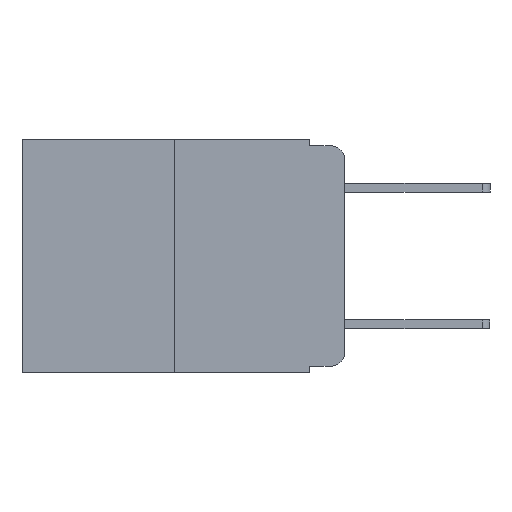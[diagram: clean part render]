
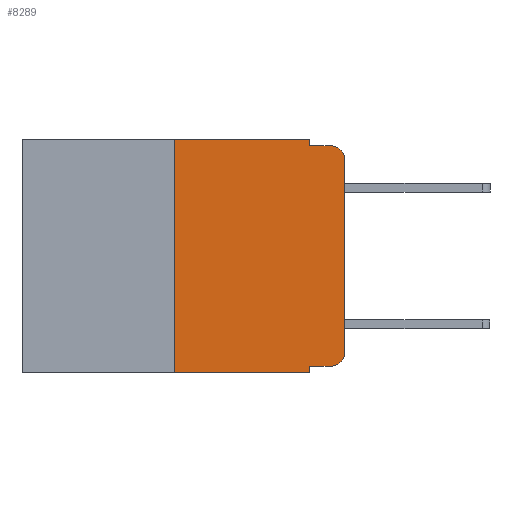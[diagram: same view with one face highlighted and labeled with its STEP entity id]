
A CAD part, left-side view. The second image highlights one B-rep face of the part: STEP entity #8289.
In plain terms, the highlighted planar face has unit normal (-1, 0, 0).
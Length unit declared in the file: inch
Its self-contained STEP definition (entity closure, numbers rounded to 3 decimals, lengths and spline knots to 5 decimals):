
#242 = EDGE_CURVE ( 'NONE', #3376, #22150, #15281, .T. ) ;
#620 = CARTESIAN_POINT ( 'NONE',  ( 0., 0.02, -0.01 ) ) ;
#632 = VECTOR ( 'NONE', #13422, 39.37008 ) ;
#712 = AXIS2_PLACEMENT_3D ( 'NONE', #9768, #23434, #2373 ) ;
#1002 = ORIENTED_EDGE ( 'NONE', *, *, #242, .F. ) ;
#1067 = VECTOR ( 'NONE', #6610, 39.37008 ) ;
#1385 = DIRECTION ( 'NONE',  ( 1., 0., 0. ) ) ;
#2243 = ORIENTED_EDGE ( 'NONE', *, *, #25216, .F. ) ;
#2373 = DIRECTION ( 'NONE',  ( 0., 0., -1. ) ) ;
#2882 = EDGE_CURVE ( 'NONE', #5389, #16315, #20441, .T. ) ;
#3294 = CARTESIAN_POINT ( 'NONE',  ( 0., 0., 0. ) ) ;
#3376 = VERTEX_POINT ( 'NONE', #22678 ) ;
#3440 = EDGE_CURVE ( 'NONE', #22150, #9264, #23692, .T. ) ;
#4256 = CARTESIAN_POINT ( 'NONE',  ( 0., 0.051, -0.343 ) ) ;
#4480 = CARTESIAN_POINT ( 'NONE',  ( 0., 0.02, -0.333 ) ) ;
#4535 = DIRECTION ( 'NONE',  ( -1., 0., 0. ) ) ;
#4758 = VECTOR ( 'NONE', #19102, 39.37008 ) ;
#5281 = DIRECTION ( 'NONE',  ( 0., 0., 1. ) ) ;
#5389 = VERTEX_POINT ( 'NONE', #19181 ) ;
#5987 = VECTOR ( 'NONE', #5281, 39.37008 ) ;
#6610 = DIRECTION ( 'NONE',  ( 0., -1., 0. ) ) ;
#6726 = AXIS2_PLACEMENT_3D ( 'NONE', #11439, #1385, #10585 ) ;
#6978 = LINE ( 'NONE', #20381, #1067 ) ;
#7067 = EDGE_CURVE ( 'NONE', #21983, #12084, #20606, .T. ) ;
#7747 = VECTOR ( 'NONE', #15739, 39.37008 ) ;
#8142 = EDGE_LOOP ( 'NONE', ( #10676, #12561, #14055, #14674, #1002, #2243, #24409, #10335, #13502, #14078 ) ) ;
#8289 = ADVANCED_FACE ( 'NONE', ( #14418 ), #19187, .F. ) ;
#8391 = CARTESIAN_POINT ( 'NONE',  ( 0., 0.25, 0. ) ) ;
#8671 = EDGE_CURVE ( 'NONE', #25123, #18181, #6978, .T. ) ;
#8984 = AXIS2_PLACEMENT_3D ( 'NONE', #16349, #4535, #18314 ) ;
#9008 = CARTESIAN_POINT ( 'NONE',  ( 0., 0.473, -0.343 ) ) ;
#9264 = VERTEX_POINT ( 'NONE', #13747 ) ;
#9768 = CARTESIAN_POINT ( 'NONE',  ( 0., 0.02, -0.03 ) ) ;
#10010 = VECTOR ( 'NONE', #19895, 39.37008 ) ;
#10024 = VERTEX_POINT ( 'NONE', #17820 ) ;
#10335 = ORIENTED_EDGE ( 'NONE', *, *, #14053, .F. ) ;
#10585 = DIRECTION ( 'NONE',  ( 0., 0., -1. ) ) ;
#10676 = ORIENTED_EDGE ( 'NONE', *, *, #17793, .T. ) ;
#11436 = CARTESIAN_POINT ( 'NONE',  ( 0., 0.051, -0.01 ) ) ;
#11439 = CARTESIAN_POINT ( 'NONE',  ( 0., 0.473, 0. ) ) ;
#12067 = CARTESIAN_POINT ( 'NONE',  ( 0., 0.051, -0.333 ) ) ;
#12084 = VERTEX_POINT ( 'NONE', #620 ) ;
#12561 = ORIENTED_EDGE ( 'NONE', *, *, #7067, .T. ) ;
#12625 = DIRECTION ( 'NONE',  ( 0., 0., -1. ) ) ;
#13263 = EDGE_CURVE ( 'NONE', #9264, #12084, #16432, .T. ) ;
#13422 = DIRECTION ( 'NONE',  ( 0., -1., 0. ) ) ;
#13502 = ORIENTED_EDGE ( 'NONE', *, *, #8671, .T. ) ;
#13579 = EDGE_CURVE ( 'NONE', #18181, #10024, #14272, .T. ) ;
#13747 = CARTESIAN_POINT ( 'NONE',  ( 0., 0.051, -0.01 ) ) ;
#13787 = CARTESIAN_POINT ( 'NONE',  ( 0., 0.051, 0. ) ) ;
#13832 = CARTESIAN_POINT ( 'NONE',  ( 0., 0.051, 0. ) ) ;
#14053 = EDGE_CURVE ( 'NONE', #25123, #16315, #23364, .T. ) ;
#14055 = ORIENTED_EDGE ( 'NONE', *, *, #13263, .F. ) ;
#14078 = ORIENTED_EDGE ( 'NONE', *, *, #13579, .T. ) ;
#14272 = CIRCLE ( 'NONE', #8984, 0.02 ) ;
#14357 = DIRECTION ( 'NONE',  ( 0., 0., 1. ) ) ;
#14418 = FACE_OUTER_BOUND ( 'NONE', #8142, .T. ) ;
#14674 = ORIENTED_EDGE ( 'NONE', *, *, #3440, .F. ) ;
#15281 = LINE ( 'NONE', #18436, #4758 ) ;
#15739 = DIRECTION ( 'NONE',  ( 0., 0., -1. ) ) ;
#15998 = VECTOR ( 'NONE', #14357, 39.37008 ) ;
#16315 = VERTEX_POINT ( 'NONE', #4256 ) ;
#16349 = CARTESIAN_POINT ( 'NONE',  ( 0., 0.02, -0.313 ) ) ;
#16432 = LINE ( 'NONE', #11436, #632 ) ;
#17731 = CARTESIAN_POINT ( 'NONE',  ( 0., 0., -0.03 ) ) ;
#17793 = EDGE_CURVE ( 'NONE', #10024, #21983, #21678, .T. ) ;
#17820 = CARTESIAN_POINT ( 'NONE',  ( 0., 0., -0.313 ) ) ;
#18181 = VERTEX_POINT ( 'NONE', #4480 ) ;
#18314 = DIRECTION ( 'NONE',  ( 0., 0., -1. ) ) ;
#18436 = CARTESIAN_POINT ( 'NONE',  ( 0., 0.473, 0. ) ) ;
#19102 = DIRECTION ( 'NONE',  ( 0., -1., 0. ) ) ;
#19181 = CARTESIAN_POINT ( 'NONE',  ( 0., 0.25, -0.343 ) ) ;
#19187 = PLANE ( 'NONE',  #6726 ) ;
#19895 = DIRECTION ( 'NONE',  ( 0., -1., 0. ) ) ;
#20270 = CARTESIAN_POINT ( 'NONE',  ( 0., 0.051, 0. ) ) ;
#20381 = CARTESIAN_POINT ( 'NONE',  ( 0., 0.051, -0.333 ) ) ;
#20441 = LINE ( 'NONE', #9008, #10010 ) ;
#20606 = CIRCLE ( 'NONE', #712, 0.02 ) ;
#21208 = LINE ( 'NONE', #8391, #15998 ) ;
#21678 = LINE ( 'NONE', #3294, #5987 ) ;
#21983 = VERTEX_POINT ( 'NONE', #17731 ) ;
#22150 = VERTEX_POINT ( 'NONE', #20270 ) ;
#22678 = CARTESIAN_POINT ( 'NONE',  ( 0., 0.25, 0. ) ) ;
#23107 = VECTOR ( 'NONE', #12625, 39.37008 ) ;
#23364 = LINE ( 'NONE', #13787, #7747 ) ;
#23434 = DIRECTION ( 'NONE',  ( -1., 0., 0. ) ) ;
#23692 = LINE ( 'NONE', #13832, #23107 ) ;
#24409 = ORIENTED_EDGE ( 'NONE', *, *, #2882, .T. ) ;
#25123 = VERTEX_POINT ( 'NONE', #12067 ) ;
#25216 = EDGE_CURVE ( 'NONE', #5389, #3376, #21208, .T. ) ;
